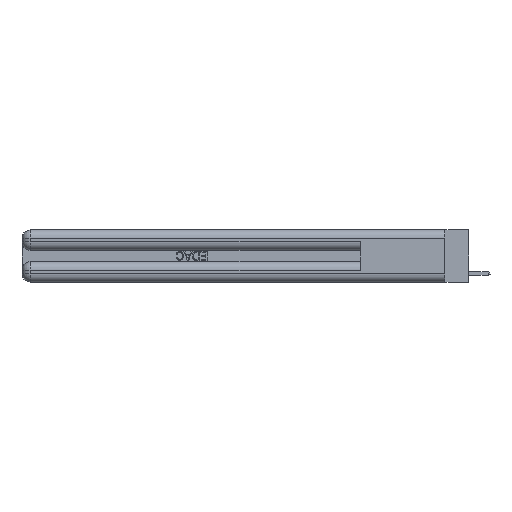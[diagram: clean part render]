
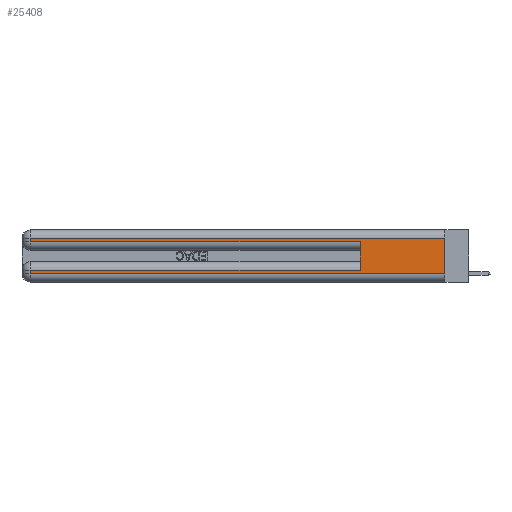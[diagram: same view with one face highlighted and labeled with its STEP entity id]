
A CAD part, left-side view. The second image highlights one B-rep face of the part: STEP entity #25408.
In plain terms, the highlighted planar face has unit normal (-1, 0, 0).
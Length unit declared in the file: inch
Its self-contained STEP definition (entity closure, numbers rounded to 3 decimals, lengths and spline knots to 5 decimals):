
#948 = CARTESIAN_POINT ( 'NONE',  ( 0., 0., 0.06 ) ) ;
#2133 = DIRECTION ( 'NONE',  ( 0., 0., 1. ) ) ;
#2211 = CARTESIAN_POINT ( 'NONE',  ( 0., 0.6, 0.085 ) ) ;
#3672 = LINE ( 'NONE', #14444, #18919 ) ;
#3684 = VERTEX_POINT ( 'NONE', #32432 ) ;
#3743 = AXIS2_PLACEMENT_3D ( 'NONE', #17683, #14498, #24775 ) ;
#3905 = CARTESIAN_POINT ( 'NONE',  ( 0., 0., 0.285 ) ) ;
#4779 = EDGE_CURVE ( 'NONE', #22402, #3684, #30276, .T. ) ;
#5325 = CARTESIAN_POINT ( 'NONE',  ( 0., 0.6, 0.145 ) ) ;
#5909 = CARTESIAN_POINT ( 'NONE',  ( 0., 0., 0.085 ) ) ;
#7129 = DIRECTION ( 'NONE',  ( 0., 0., -1. ) ) ;
#7584 = VERTEX_POINT ( 'NONE', #18985 ) ;
#9761 = PLANE ( 'NONE',  #3743 ) ;
#10139 = CARTESIAN_POINT ( 'NONE',  ( 0., 0., 0.31 ) ) ;
#10645 = DIRECTION ( 'NONE',  ( 0., 0., -1. ) ) ;
#10760 = EDGE_CURVE ( 'NONE', #16048, #24135, #19308, .T. ) ;
#13452 = CARTESIAN_POINT ( 'NONE',  ( 0., 2.94, 0.06 ) ) ;
#13589 = DIRECTION ( 'NONE',  ( 0., -1., 0. ) ) ;
#14007 = ORIENTED_EDGE ( 'NONE', *, *, #16132, .F. ) ;
#14444 = CARTESIAN_POINT ( 'NONE',  ( 0., 0., 0.37 ) ) ;
#14498 = DIRECTION ( 'NONE',  ( 1., 0., 0. ) ) ;
#14788 = ORIENTED_EDGE ( 'NONE', *, *, #19399, .T. ) ;
#15023 = ORIENTED_EDGE ( 'NONE', *, *, #17486, .T. ) ;
#16048 = VERTEX_POINT ( 'NONE', #13452 ) ;
#16132 = EDGE_CURVE ( 'NONE', #32608, #24135, #3672, .T. ) ;
#16974 = DIRECTION ( 'NONE',  ( 0., 0., -1. ) ) ;
#17287 = CARTESIAN_POINT ( 'NONE',  ( 0., 2.94, 0.31 ) ) ;
#17486 = EDGE_CURVE ( 'NONE', #22402, #25757, #29162, .T. ) ;
#17683 = CARTESIAN_POINT ( 'NONE',  ( 0., 0., 0.37 ) ) ;
#18919 = VECTOR ( 'NONE', #16974, 39.37008 ) ;
#18985 = CARTESIAN_POINT ( 'NONE',  ( 0., 2.94, 0.285 ) ) ;
#19215 = VECTOR ( 'NONE', #2133, 39.37008 ) ;
#19283 = EDGE_CURVE ( 'NONE', #26391, #7584, #22293, .T. ) ;
#19308 = LINE ( 'NONE', #948, #29194 ) ;
#19399 = EDGE_CURVE ( 'NONE', #32608, #26391, #33062, .T. ) ;
#19620 = CARTESIAN_POINT ( 'NONE',  ( 0., 2.94, 0.37 ) ) ;
#19647 = EDGE_CURVE ( 'NONE', #7584, #3684, #19897, .T. ) ;
#19897 = LINE ( 'NONE', #3905, #31668 ) ;
#20156 = CARTESIAN_POINT ( 'NONE',  ( 0., 2.94, 0.085 ) ) ;
#20426 = DIRECTION ( 'NONE',  ( 0., 1., 0. ) ) ;
#21353 = ORIENTED_EDGE ( 'NONE', *, *, #19283, .T. ) ;
#22293 = LINE ( 'NONE', #19620, #28434 ) ;
#22402 = VERTEX_POINT ( 'NONE', #2211 ) ;
#24135 = VERTEX_POINT ( 'NONE', #24595 ) ;
#24359 = ORIENTED_EDGE ( 'NONE', *, *, #25888, .T. ) ;
#24595 = CARTESIAN_POINT ( 'NONE',  ( 0., 0., 0.06 ) ) ;
#24693 = VECTOR ( 'NONE', #20426, 39.37008 ) ;
#24775 = DIRECTION ( 'NONE',  ( 0., 0., -1. ) ) ;
#25408 = ADVANCED_FACE ( 'NONE', ( #32842 ), #9761, .F. ) ;
#25731 = CARTESIAN_POINT ( 'NONE',  ( 0., 0., 0.31 ) ) ;
#25757 = VERTEX_POINT ( 'NONE', #20156 ) ;
#25888 = EDGE_CURVE ( 'NONE', #25757, #16048, #31032, .T. ) ;
#26391 = VERTEX_POINT ( 'NONE', #17287 ) ;
#26468 = DIRECTION ( 'NONE',  ( 0., 1., 0. ) ) ;
#28434 = VECTOR ( 'NONE', #7129, 39.37008 ) ;
#28508 = VECTOR ( 'NONE', #10645, 39.37008 ) ;
#28857 = ORIENTED_EDGE ( 'NONE', *, *, #4779, .F. ) ;
#29162 = LINE ( 'NONE', #5909, #33219 ) ;
#29185 = CARTESIAN_POINT ( 'NONE',  ( 0., 2.94, 0.37 ) ) ;
#29194 = VECTOR ( 'NONE', #13589, 39.37008 ) ;
#29504 = DIRECTION ( 'NONE',  ( 0., -1., 0. ) ) ;
#29795 = ORIENTED_EDGE ( 'NONE', *, *, #10760, .T. ) ;
#30276 = LINE ( 'NONE', #5325, #19215 ) ;
#30967 = EDGE_LOOP ( 'NONE', ( #14007, #14788, #21353, #32193, #28857, #15023, #24359, #29795 ) ) ;
#31032 = LINE ( 'NONE', #29185, #28508 ) ;
#31668 = VECTOR ( 'NONE', #29504, 39.37008 ) ;
#32193 = ORIENTED_EDGE ( 'NONE', *, *, #19647, .T. ) ;
#32432 = CARTESIAN_POINT ( 'NONE',  ( 0., 0.6, 0.285 ) ) ;
#32608 = VERTEX_POINT ( 'NONE', #25731 ) ;
#32842 = FACE_OUTER_BOUND ( 'NONE', #30967, .T. ) ;
#33062 = LINE ( 'NONE', #10139, #24693 ) ;
#33219 = VECTOR ( 'NONE', #26468, 39.37008 ) ;
